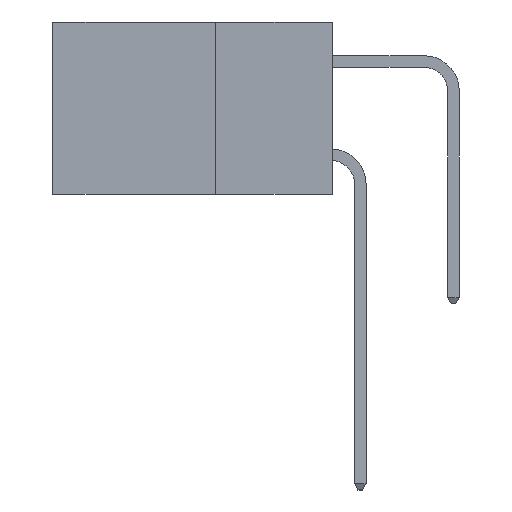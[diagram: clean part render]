
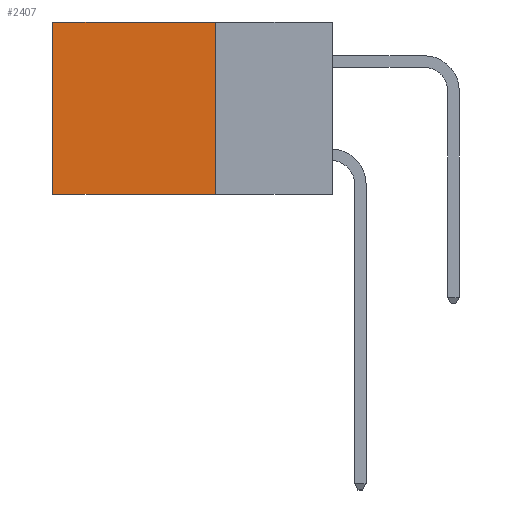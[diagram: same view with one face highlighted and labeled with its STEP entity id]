
A CAD part, left-side view. The second image highlights one B-rep face of the part: STEP entity #2407.
In plain terms, the highlighted planar face has unit normal (-1, 0, 0).
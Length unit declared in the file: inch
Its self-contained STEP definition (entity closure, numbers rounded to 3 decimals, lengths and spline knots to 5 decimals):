
#407 = EDGE_CURVE ( 'NONE', #4485, #2607, #4670, .T. ) ;
#864 = ORIENTED_EDGE ( 'NONE', *, *, #2340, .T. ) ;
#1097 = CARTESIAN_POINT ( 'NONE',  ( 0.2615, 0.25, -0.37 ) ) ;
#1102 = DIRECTION ( 'NONE',  ( 0., 1., 0. ) ) ;
#1325 = AXIS2_PLACEMENT_3D ( 'NONE', #9463, #9359, #9283 ) ;
#1490 = VECTOR ( 'NONE', #11614, 39.37008 ) ;
#1928 = LINE ( 'NONE', #11574, #1490 ) ;
#1933 = VERTEX_POINT ( 'NONE', #14088 ) ;
#2340 = EDGE_CURVE ( 'NONE', #1933, #4679, #1928, .T. ) ;
#2407 = ADVANCED_FACE ( 'NONE', ( #13293 ), #9414, .F. ) ;
#2607 = VERTEX_POINT ( 'NONE', #5893 ) ;
#3449 = EDGE_LOOP ( 'NONE', ( #864, #4734, #11884, #3843 ) ) ;
#3777 = CARTESIAN_POINT ( 'NONE',  ( 0.2615, 0.25, 0. ) ) ;
#3843 = ORIENTED_EDGE ( 'NONE', *, *, #5206, .T. ) ;
#3857 = DIRECTION ( 'NONE',  ( 0., 1., 0. ) ) ;
#4485 = VERTEX_POINT ( 'NONE', #12045 ) ;
#4670 = LINE ( 'NONE', #13827, #11037 ) ;
#4679 = VERTEX_POINT ( 'NONE', #9649 ) ;
#4734 = ORIENTED_EDGE ( 'NONE', *, *, #13873, .F. ) ;
#5206 = EDGE_CURVE ( 'NONE', #4485, #1933, #7267, .T. ) ;
#5893 = CARTESIAN_POINT ( 'NONE',  ( 0.2615, 0.25, -0.37 ) ) ;
#6627 = LINE ( 'NONE', #1097, #12922 ) ;
#7267 = LINE ( 'NONE', #3777, #13550 ) ;
#9283 = DIRECTION ( 'NONE',  ( 0., 0., -1. ) ) ;
#9359 = DIRECTION ( 'NONE',  ( 1., 0., 0. ) ) ;
#9414 = PLANE ( 'NONE',  #1325 ) ;
#9463 = CARTESIAN_POINT ( 'NONE',  ( 0.2615, 0.25, -0.37 ) ) ;
#9649 = CARTESIAN_POINT ( 'NONE',  ( 0.2615, 0.6, -0.37 ) ) ;
#11037 = VECTOR ( 'NONE', #13048, 39.37008 ) ;
#11574 = CARTESIAN_POINT ( 'NONE',  ( 0.2615, 0.6, -0.37 ) ) ;
#11614 = DIRECTION ( 'NONE',  ( 0., 0., -1. ) ) ;
#11884 = ORIENTED_EDGE ( 'NONE', *, *, #407, .F. ) ;
#12045 = CARTESIAN_POINT ( 'NONE',  ( 0.2615, 0.25, 0. ) ) ;
#12922 = VECTOR ( 'NONE', #1102, 39.37008 ) ;
#13048 = DIRECTION ( 'NONE',  ( 0., 0., -1. ) ) ;
#13293 = FACE_OUTER_BOUND ( 'NONE', #3449, .T. ) ;
#13550 = VECTOR ( 'NONE', #3857, 39.37008 ) ;
#13827 = CARTESIAN_POINT ( 'NONE',  ( 0.2615, 0.25, -0.37 ) ) ;
#13873 = EDGE_CURVE ( 'NONE', #2607, #4679, #6627, .T. ) ;
#14088 = CARTESIAN_POINT ( 'NONE',  ( 0.2615, 0.6, 0. ) ) ;
